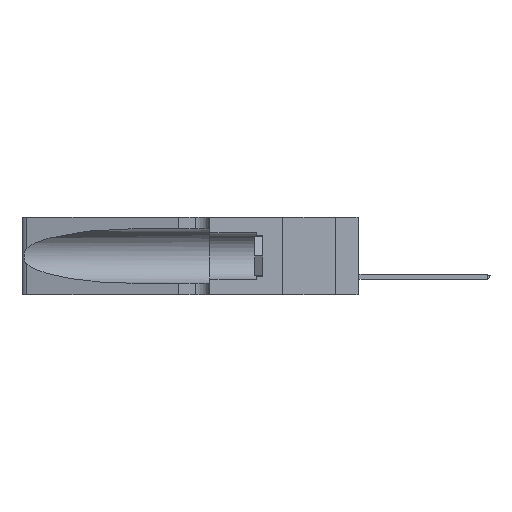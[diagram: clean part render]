
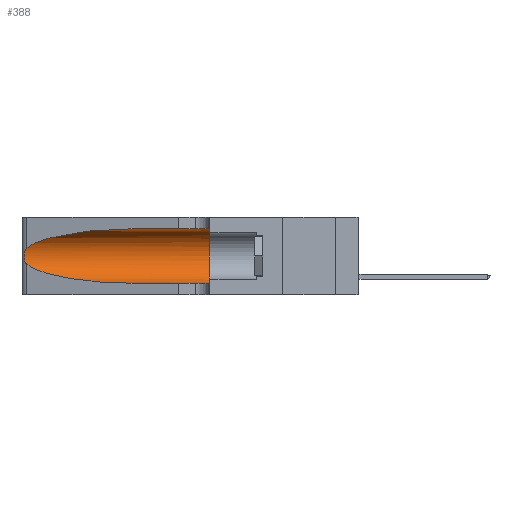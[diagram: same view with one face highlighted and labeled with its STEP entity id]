
A CAD part, left-side view. The second image highlights one B-rep face of the part: STEP entity #388.
In plain terms, the highlighted cylindrical face has radius 3.308 mm (diameter 6.617 mm), a partial arc.
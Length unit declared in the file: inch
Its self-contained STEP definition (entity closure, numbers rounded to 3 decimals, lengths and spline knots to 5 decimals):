
#388 = ADVANCED_FACE ( 'NONE', ( #8065 ), #37656, .F. ) ;
#542 = EDGE_CURVE ( 'NONE', #13930, #24220, #22869, .T. ) ;
#755 = CARTESIAN_POINT ( 'NONE',  ( 0.25487, 1.22718, 0.22369 ) ) ;
#893 = CARTESIAN_POINT ( 'NONE',  ( 0.26075, 1.23896, 0.19203 ) ) ;
#1782 = CARTESIAN_POINT ( 'NONE',  ( 0.1305, 0.72297, 0.05475 ) ) ;
#1960 = CARTESIAN_POINT ( 'NONE',  ( 0.1305, 0.72297, 0.05475 ) ) ;
#2633 = CARTESIAN_POINT ( 'NONE',  ( 0.1305, 1.61858, 0.31525 ) ) ;
#3266 = ORIENTED_EDGE ( 'NONE', *, *, #22382, .T. ) ;
#4443 = EDGE_CURVE ( 'NONE', #21037, #21902, #33852, .T. ) ;
#6742 = DIRECTION ( 'NONE',  ( 0., -1., 0. ) ) ;
#7141 = CARTESIAN_POINT ( 'NONE',  ( 0.26075, 1.23896, 0.178 ) ) ;
#8065 = FACE_OUTER_BOUND ( 'NONE', #18026, .T. ) ;
#8673 = AXIS2_PLACEMENT_3D ( 'NONE', #9215, #34673, #37845 ) ;
#9215 = CARTESIAN_POINT ( 'NONE',  ( 0.1305, 0.35, 0.185 ) ) ;
#9605 = VECTOR ( 'NONE', #10798, 39.37008 ) ;
#10271 = ORIENTED_EDGE ( 'NONE', *, *, #542, .T. ) ;
#10429 = AXIS2_PLACEMENT_3D ( 'NONE', #36809, #27346, #30493 ) ;
#10798 = DIRECTION ( 'NONE',  ( 0., -1., 0. ) ) ;
#11767 =( BOUNDED_CURVE ( )  B_SPLINE_CURVE ( 3, ( #13961, #35989, #26968, #1782 ),
 .UNSPECIFIED., .F., .F. ) 
 B_SPLINE_CURVE_WITH_KNOTS ( ( 4, 4 ),
 ( 3.44316, 4.71239 ),
 .UNSPECIFIED. ) 
 CURVE ( )  GEOMETRIC_REPRESENTATION_ITEM ( )  RATIONAL_B_SPLINE_CURVE ( ( 1., 0.87, 0.87, 1. ) ) 
 REPRESENTATION_ITEM ( '' )  );
#13361 = CARTESIAN_POINT ( 'NONE',  ( 0.25854, 1.2359, 0.20912 ) ) ;
#13753 = CARTESIAN_POINT ( 'NONE',  ( 0.25789, 1.23486, 0.15765 ) ) ;
#13930 = VERTEX_POINT ( 'NONE', #19364 ) ;
#13961 = CARTESIAN_POINT ( 'NONE',  ( 0.25487, 1.22718, 0.14631 ) ) ;
#16260 = CARTESIAN_POINT ( 'NONE',  ( 0.25787, 1.23484, 0.2124 ) ) ;
#18026 = EDGE_LOOP ( 'NONE', ( #40259, #10271, #32834, #3266, #26982, #32661 ) ) ;
#18272 = VERTEX_POINT ( 'NONE', #1960 ) ;
#19055 =( BOUNDED_CURVE ( )  B_SPLINE_CURVE ( 3, ( #39372, #26878, #39929, #21722 ),
 .UNSPECIFIED., .F., .T. ) 
 B_SPLINE_CURVE_WITH_KNOTS ( ( 4, 4 ),
 ( 1.5708, 2.84003 ),
 .UNSPECIFIED. ) 
 CURVE ( )  GEOMETRIC_REPRESENTATION_ITEM ( )  RATIONAL_B_SPLINE_CURVE ( ( 1., 0.87, 0.87, 1. ) ) 
 REPRESENTATION_ITEM ( '' )  );
#19364 = CARTESIAN_POINT ( 'NONE',  ( 0.25487, 1.22718, 0.22369 ) ) ;
#19465 = CARTESIAN_POINT ( 'NONE',  ( 0.1305, 0.35, 0.05475 ) ) ;
#19851 = CARTESIAN_POINT ( 'NONE',  ( 0.25639, 1.23186, 0.15144 ) ) ;
#20549 = EDGE_CURVE ( 'NONE', #21037, #13930, #19055, .T. ) ;
#21037 = VERTEX_POINT ( 'NONE', #30457 ) ;
#21722 = CARTESIAN_POINT ( 'NONE',  ( 0.25487, 1.22718, 0.22369 ) ) ;
#21902 = VERTEX_POINT ( 'NONE', #33126 ) ;
#22382 = EDGE_CURVE ( 'NONE', #18272, #36337, #35676, .T. ) ;
#22869 = B_SPLINE_CURVE_WITH_KNOTS ( 'NONE', 3,
 ( #755, #28685, #31978, #16260, #13361, #29774, #893, #7141, #29488, #35520, #13753, #19851, #38961, #39109 ),
 .UNSPECIFIED., .F., .F.,
 ( 4, 2, 2, 2, 2, 2, 4 ),
 ( 0., 0.00027, 0.00053, 0.00107, 0.0016, 0.00187, 0.00214 ),
 .UNSPECIFIED. ) ;
#24220 = VERTEX_POINT ( 'NONE', #38923 ) ;
#25976 = VECTOR ( 'NONE', #6742, 39.37008 ) ;
#26522 = CARTESIAN_POINT ( 'NONE',  ( 0.1305, 1.61858, 0.05475 ) ) ;
#26878 = CARTESIAN_POINT ( 'NONE',  ( 0.18966, 0.96281, 0.31525 ) ) ;
#26968 = CARTESIAN_POINT ( 'NONE',  ( 0.18966, 0.96281, 0.05475 ) ) ;
#26982 = ORIENTED_EDGE ( 'NONE', *, *, #38003, .F. ) ;
#27346 = DIRECTION ( 'NONE',  ( 0., -1., 0. ) ) ;
#28685 = CARTESIAN_POINT ( 'NONE',  ( 0.25555, 1.22994, 0.2215 ) ) ;
#29488 = CARTESIAN_POINT ( 'NONE',  ( 0.26017, 1.23833, 0.17102 ) ) ;
#29774 = CARTESIAN_POINT ( 'NONE',  ( 0.26018, 1.23835, 0.19895 ) ) ;
#30457 = CARTESIAN_POINT ( 'NONE',  ( 0.1305, 0.72297, 0.31525 ) ) ;
#30493 = DIRECTION ( 'NONE',  ( 0., 0., -1. ) ) ;
#31978 = CARTESIAN_POINT ( 'NONE',  ( 0.25639, 1.23184, 0.21858 ) ) ;
#32661 = ORIENTED_EDGE ( 'NONE', *, *, #4443, .F. ) ;
#32834 = ORIENTED_EDGE ( 'NONE', *, *, #38838, .T. ) ;
#33126 = CARTESIAN_POINT ( 'NONE',  ( 0.1305, 0.35, 0.31525 ) ) ;
#33852 = LINE ( 'NONE', #2633, #25976 ) ;
#34673 = DIRECTION ( 'NONE',  ( 0., 1., 0. ) ) ;
#35520 = CARTESIAN_POINT ( 'NONE',  ( 0.25856, 1.23593, 0.16098 ) ) ;
#35676 = LINE ( 'NONE', #26522, #9605 ) ;
#35989 = CARTESIAN_POINT ( 'NONE',  ( 0.2373, 1.15595, 0.08982 ) ) ;
#36337 = VERTEX_POINT ( 'NONE', #19465 ) ;
#36809 = CARTESIAN_POINT ( 'NONE',  ( 0.1305, 1.61858, 0.185 ) ) ;
#37656 = CYLINDRICAL_SURFACE ( 'NONE', #10429, 0.13025 ) ;
#37845 = DIRECTION ( 'NONE',  ( 0., 0., 1. ) ) ;
#38003 = EDGE_CURVE ( 'NONE', #21902, #36337, #40060, .T. ) ;
#38838 = EDGE_CURVE ( 'NONE', #24220, #18272, #11767, .T. ) ;
#38923 = CARTESIAN_POINT ( 'NONE',  ( 0.25487, 1.22718, 0.14631 ) ) ;
#38961 = CARTESIAN_POINT ( 'NONE',  ( 0.25555, 1.22993, 0.14849 ) ) ;
#39109 = CARTESIAN_POINT ( 'NONE',  ( 0.25487, 1.22718, 0.14631 ) ) ;
#39372 = CARTESIAN_POINT ( 'NONE',  ( 0.1305, 0.72297, 0.31525 ) ) ;
#39929 = CARTESIAN_POINT ( 'NONE',  ( 0.2373, 1.15595, 0.28018 ) ) ;
#40060 = CIRCLE ( 'NONE', #8673, 0.13025 ) ;
#40259 = ORIENTED_EDGE ( 'NONE', *, *, #20549, .T. ) ;
